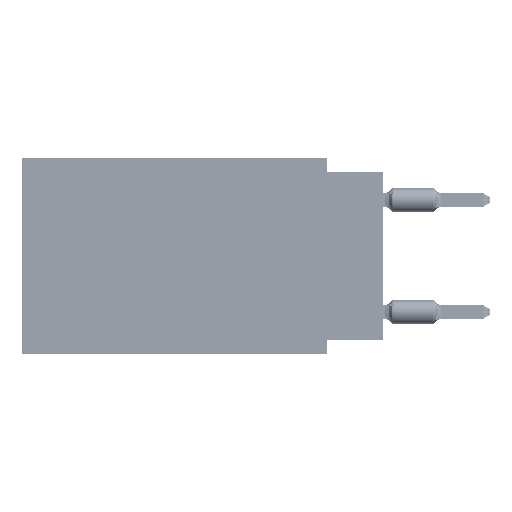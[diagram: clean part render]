
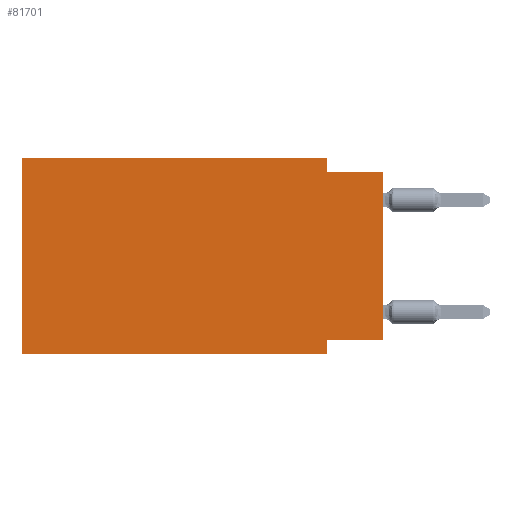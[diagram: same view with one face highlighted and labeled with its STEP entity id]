
A CAD part, left-side view. The second image highlights one B-rep face of the part: STEP entity #81701.
In plain terms, the highlighted planar face has unit normal (-1, 0, 0).
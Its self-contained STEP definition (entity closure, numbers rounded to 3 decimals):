
#3408 = DIRECTION ( 'NONE',  ( 0., 0., -1. ) ) ;
#4184 = VERTEX_POINT ( 'NONE', #103941 ) ;
#4859 = LINE ( 'NONE', #6689, #52724 ) ;
#6490 = CARTESIAN_POINT ( 'NONE',  ( 0., 2.54, 0. ) ) ;
#6689 = CARTESIAN_POINT ( 'NONE',  ( 0., 16.383, 0. ) ) ;
#7810 = CARTESIAN_POINT ( 'NONE',  ( 0., 0., -0.635 ) ) ;
#8263 = CARTESIAN_POINT ( 'NONE',  ( 0., 2.54, -8.89 ) ) ;
#9795 = EDGE_CURVE ( 'NONE', #33795, #94915, #4859, .T. ) ;
#11083 = VECTOR ( 'NONE', #30848, 1000. ) ;
#11352 = CARTESIAN_POINT ( 'NONE',  ( 0., 16.383, -8.89 ) ) ;
#14029 = CARTESIAN_POINT ( 'NONE',  ( 0., 16.383, 0. ) ) ;
#14210 = ORIENTED_EDGE ( 'NONE', *, *, #61903, .T. ) ;
#14608 = VECTOR ( 'NONE', #54724, 1000. ) ;
#16551 = DIRECTION ( 'NONE',  ( 0., 0., 1. ) ) ;
#17012 = VECTOR ( 'NONE', #86883, 1000. ) ;
#17018 = VERTEX_POINT ( 'NONE', #115248 ) ;
#18468 = EDGE_CURVE ( 'NONE', #55453, #115003, #38206, .T. ) ;
#28122 = DIRECTION ( 'NONE',  ( 0., -1., 0. ) ) ;
#29564 = VERTEX_POINT ( 'NONE', #86070 ) ;
#30848 = DIRECTION ( 'NONE',  ( 0., -1., 0. ) ) ;
#30925 = ORIENTED_EDGE ( 'NONE', *, *, #86637, .F. ) ;
#33795 = VERTEX_POINT ( 'NONE', #11352 ) ;
#35398 = CARTESIAN_POINT ( 'NONE',  ( 0., 16.383, 0. ) ) ;
#38206 = LINE ( 'NONE', #46822, #108662 ) ;
#39823 = CARTESIAN_POINT ( 'NONE',  ( 0., 0., -8.255 ) ) ;
#41143 = FACE_OUTER_BOUND ( 'NONE', #50834, .T. ) ;
#43591 = DIRECTION ( 'NONE',  ( 0., 0., -1. ) ) ;
#45193 = CARTESIAN_POINT ( 'NONE',  ( 0., 16.383, 0. ) ) ;
#45399 = LINE ( 'NONE', #7810, #100115 ) ;
#46822 = CARTESIAN_POINT ( 'NONE',  ( 0., 2.54, -8.89 ) ) ;
#50834 = EDGE_LOOP ( 'NONE', ( #104017, #117429, #86871, #68393, #76593, #14210, #59890, #30925 ) ) ;
#52724 = VECTOR ( 'NONE', #16551, 1000. ) ;
#54724 = DIRECTION ( 'NONE',  ( 0., 0., 1. ) ) ;
#54827 = AXIS2_PLACEMENT_3D ( 'NONE', #14029, #88554, #43591 ) ;
#55453 = VERTEX_POINT ( 'NONE', #62726 ) ;
#59890 = ORIENTED_EDGE ( 'NONE', *, *, #18468, .F. ) ;
#61871 = EDGE_CURVE ( 'NONE', #94915, #88521, #119771, .T. ) ;
#61903 = EDGE_CURVE ( 'NONE', #33795, #115003, #82810, .T. ) ;
#62726 = CARTESIAN_POINT ( 'NONE',  ( 0., 2.54, -8.255 ) ) ;
#68393 = ORIENTED_EDGE ( 'NONE', *, *, #61871, .F. ) ;
#76593 = ORIENTED_EDGE ( 'NONE', *, *, #9795, .F. ) ;
#79209 = LINE ( 'NONE', #39823, #106770 ) ;
#81701 = ADVANCED_FACE ( 'NONE', ( #41143 ), #116880, .F. ) ;
#81871 = EDGE_CURVE ( 'NONE', #29564, #17018, #45399, .T. ) ;
#82810 = LINE ( 'NONE', #115206, #11083 ) ;
#83668 = LINE ( 'NONE', #100935, #14608 ) ;
#85991 = CARTESIAN_POINT ( 'NONE',  ( 0., 2.54, 0. ) ) ;
#86070 = CARTESIAN_POINT ( 'NONE',  ( 0., 2.54, -0.635 ) ) ;
#86637 = EDGE_CURVE ( 'NONE', #4184, #55453, #79209, .T. ) ;
#86871 = ORIENTED_EDGE ( 'NONE', *, *, #109352, .F. ) ;
#86883 = DIRECTION ( 'NONE',  ( 0., -1., 0. ) ) ;
#88521 = VERTEX_POINT ( 'NONE', #6490 ) ;
#88554 = DIRECTION ( 'NONE',  ( 1., 0., 0. ) ) ;
#94915 = VERTEX_POINT ( 'NONE', #45193 ) ;
#95844 = LINE ( 'NONE', #85991, #98120 ) ;
#98120 = VECTOR ( 'NONE', #3408, 1000. ) ;
#100115 = VECTOR ( 'NONE', #28122, 1000. ) ;
#100935 = CARTESIAN_POINT ( 'NONE',  ( 0., 0., 0. ) ) ;
#103941 = CARTESIAN_POINT ( 'NONE',  ( 0., 0., -8.255 ) ) ;
#104017 = ORIENTED_EDGE ( 'NONE', *, *, #121020, .T. ) ;
#106770 = VECTOR ( 'NONE', #114338, 1000. ) ;
#108662 = VECTOR ( 'NONE', #112720, 1000. ) ;
#109352 = EDGE_CURVE ( 'NONE', #88521, #29564, #95844, .T. ) ;
#112720 = DIRECTION ( 'NONE',  ( 0., 0., -1. ) ) ;
#114338 = DIRECTION ( 'NONE',  ( 0., 1., 0. ) ) ;
#115003 = VERTEX_POINT ( 'NONE', #8263 ) ;
#115206 = CARTESIAN_POINT ( 'NONE',  ( 0., 16.383, -8.89 ) ) ;
#115248 = CARTESIAN_POINT ( 'NONE',  ( 0., 0., -0.635 ) ) ;
#116880 = PLANE ( 'NONE',  #54827 ) ;
#117429 = ORIENTED_EDGE ( 'NONE', *, *, #81871, .F. ) ;
#119771 = LINE ( 'NONE', #35398, #17012 ) ;
#121020 = EDGE_CURVE ( 'NONE', #4184, #17018, #83668, .T. ) ;
